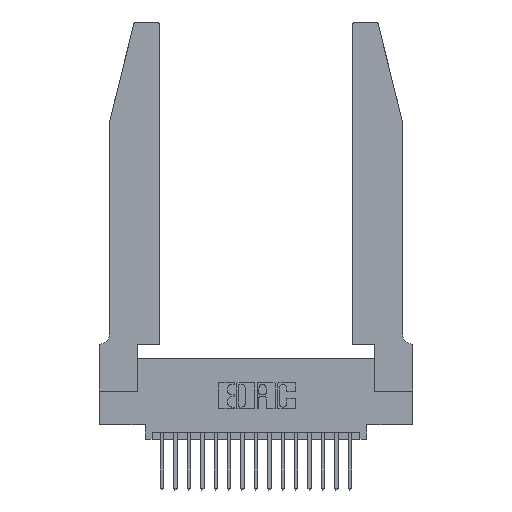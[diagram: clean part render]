
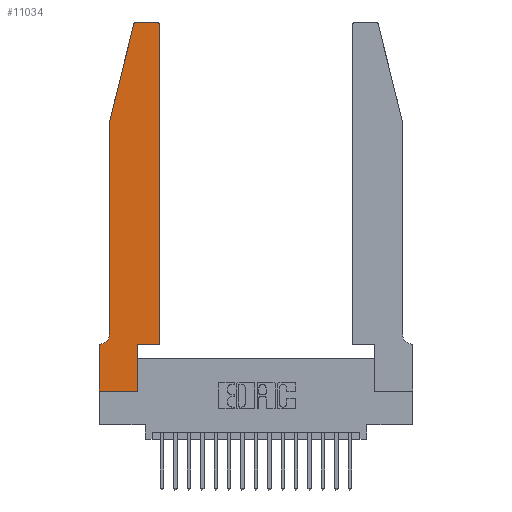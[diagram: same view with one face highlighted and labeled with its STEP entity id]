
A CAD part, top view. The second image highlights one B-rep face of the part: STEP entity #11034.
In plain terms, the highlighted planar face has unit normal (0, 0, 1).
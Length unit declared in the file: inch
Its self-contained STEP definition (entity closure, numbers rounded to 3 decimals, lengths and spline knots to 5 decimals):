
#101 = VERTEX_POINT ( 'NONE', #10746 ) ;
#145 = CARTESIAN_POINT ( 'NONE',  ( 0.4505, 2.72, 0.37 ) ) ;
#153 = ORIENTED_EDGE ( 'NONE', *, *, #16414, .T. ) ;
#239 = DIRECTION ( 'NONE',  ( -0.239, -0.971, 0. ) ) ;
#308 = DIRECTION ( 'NONE',  ( 0., 0., 1. ) ) ;
#539 = VECTOR ( 'NONE', #10012, 39.37008 ) ;
#1547 = ORIENTED_EDGE ( 'NONE', *, *, #12111, .T. ) ;
#1952 = CARTESIAN_POINT ( 'NONE',  ( 0.4505, 0.35, 0.37 ) ) ;
#1962 = VERTEX_POINT ( 'NONE', #7361 ) ;
#2054 = CIRCLE ( 'NONE', #19312, 0.03 ) ;
#2263 = DIRECTION ( 'NONE',  ( -1., 0., 0. ) ) ;
#2495 = LINE ( 'NONE', #17191, #10495 ) ;
#2787 = VECTOR ( 'NONE', #11345, 39.37008 ) ;
#3312 = LINE ( 'NONE', #6693, #2787 ) ;
#3370 = FACE_OUTER_BOUND ( 'NONE', #5832, .T. ) ;
#3449 = CIRCLE ( 'NONE', #17180, 0.07 ) ;
#3873 = EDGE_CURVE ( 'NONE', #7588, #11189, #2495, .T. ) ;
#3948 = ORIENTED_EDGE ( 'NONE', *, *, #14976, .T. ) ;
#4078 = VERTEX_POINT ( 'NONE', #8341 ) ;
#4102 = EDGE_CURVE ( 'NONE', #9212, #4964, #17397, .T. ) ;
#4835 = AXIS2_PLACEMENT_3D ( 'NONE', #15529, #17072, #7827 ) ;
#4964 = VERTEX_POINT ( 'NONE', #13429 ) ;
#5278 = VERTEX_POINT ( 'NONE', #145 ) ;
#5389 = CARTESIAN_POINT ( 'NONE',  ( 0.4505, 0.35, 0.37 ) ) ;
#5608 = CARTESIAN_POINT ( 'NONE',  ( 0.0755, 0.35, 0.37 ) ) ;
#5832 = EDGE_LOOP ( 'NONE', ( #7102, #153, #7049, #10660, #3948, #7338, #12381, #1547, #9875, #10786, #15272, #8742 ) ) ;
#5968 = VECTOR ( 'NONE', #2263, 39.37008 ) ;
#6265 = PLANE ( 'NONE',  #4835 ) ;
#6290 = VERTEX_POINT ( 'NONE', #16852 ) ;
#6476 = LINE ( 'NONE', #5608, #5968 ) ;
#6651 = CARTESIAN_POINT ( 'NONE',  ( 0.284, 2.72, 0.37 ) ) ;
#6693 = CARTESIAN_POINT ( 'NONE',  ( 0.2605, 2.75, 0.37 ) ) ;
#6741 = CIRCLE ( 'NONE', #8019, 0.03 ) ;
#7032 = DIRECTION ( 'NONE',  ( 1., 0., 0. ) ) ;
#7049 = ORIENTED_EDGE ( 'NONE', *, *, #9142, .T. ) ;
#7102 = ORIENTED_EDGE ( 'NONE', *, *, #12440, .T. ) ;
#7338 = ORIENTED_EDGE ( 'NONE', *, *, #10852, .T. ) ;
#7361 = CARTESIAN_POINT ( 'NONE',  ( 0.4205, 2.75, 0.37 ) ) ;
#7459 = DIRECTION ( 'NONE',  ( 1., 0., 0. ) ) ;
#7588 = VERTEX_POINT ( 'NONE', #9955 ) ;
#7590 = CARTESIAN_POINT ( 'NONE',  ( 0.0055, 0.42, 0.37 ) ) ;
#7827 = DIRECTION ( 'NONE',  ( 1., 0., 0. ) ) ;
#7936 = VECTOR ( 'NONE', #7032, 39.37008 ) ;
#8019 = AXIS2_PLACEMENT_3D ( 'NONE', #6651, #17466, #8211 ) ;
#8211 = DIRECTION ( 'NONE',  ( 1., 0., 0. ) ) ;
#8341 = CARTESIAN_POINT ( 'NONE',  ( 0.0055, 0.35, 0.37 ) ) ;
#8392 = CARTESIAN_POINT ( 'NONE',  ( 0.0755, 2., 0.37 ) ) ;
#8549 = EDGE_CURVE ( 'NONE', #16070, #5278, #16534, .T. ) ;
#8742 = ORIENTED_EDGE ( 'NONE', *, *, #19564, .T. ) ;
#8851 = LINE ( 'NONE', #11962, #16584 ) ;
#8934 = EDGE_CURVE ( 'NONE', #14857, #16331, #16998, .T. ) ;
#9135 = DIRECTION ( 'NONE',  ( -1., 0., 0. ) ) ;
#9142 = EDGE_CURVE ( 'NONE', #6290, #14857, #18186, .T. ) ;
#9212 = VERTEX_POINT ( 'NONE', #19320 ) ;
#9424 = CARTESIAN_POINT ( 'NONE',  ( 0.0755, 0.42, 0.37 ) ) ;
#9875 = ORIENTED_EDGE ( 'NONE', *, *, #4102, .T. ) ;
#9955 = CARTESIAN_POINT ( 'NONE',  ( 0., 0.35, 0.37 ) ) ;
#9995 = CARTESIAN_POINT ( 'NONE',  ( 0.4205, 2.72, 0.37 ) ) ;
#10012 = DIRECTION ( 'NONE',  ( 0., 1., 0. ) ) ;
#10308 = CARTESIAN_POINT ( 'NONE',  ( 0.4505, 0.35, 0.37 ) ) ;
#10495 = VECTOR ( 'NONE', #18685, 39.37008 ) ;
#10660 = ORIENTED_EDGE ( 'NONE', *, *, #8934, .T. ) ;
#10746 = CARTESIAN_POINT ( 'NONE',  ( 0.284, 2.75, 0.37 ) ) ;
#10765 = EDGE_CURVE ( 'NONE', #4964, #16070, #12025, .T. ) ;
#10786 = ORIENTED_EDGE ( 'NONE', *, *, #10765, .T. ) ;
#10852 = EDGE_CURVE ( 'NONE', #4078, #7588, #6476, .T. ) ;
#11034 = ADVANCED_FACE ( 'NONE', ( #3370 ), #6265, .T. ) ;
#11189 = VERTEX_POINT ( 'NONE', #12735 ) ;
#11345 = DIRECTION ( 'NONE',  ( -1., 0., 0. ) ) ;
#11552 = DIRECTION ( 'NONE',  ( 1., 0., 0. ) ) ;
#11927 = VECTOR ( 'NONE', #14642, 39.37008 ) ;
#11962 = CARTESIAN_POINT ( 'NONE',  ( 0., 0., 0.37 ) ) ;
#12025 = LINE ( 'NONE', #5389, #7936 ) ;
#12111 = EDGE_CURVE ( 'NONE', #11189, #9212, #8851, .T. ) ;
#12381 = ORIENTED_EDGE ( 'NONE', *, *, #3873, .T. ) ;
#12440 = EDGE_CURVE ( 'NONE', #1962, #101, #3312, .T. ) ;
#12735 = CARTESIAN_POINT ( 'NONE',  ( 0., 0., 0.37 ) ) ;
#12876 = VECTOR ( 'NONE', #17248, 39.37008 ) ;
#13382 = CARTESIAN_POINT ( 'NONE',  ( 0.0755, 2., 0.37 ) ) ;
#13429 = CARTESIAN_POINT ( 'NONE',  ( 0.2865, 0.35, 0.37 ) ) ;
#14076 = VECTOR ( 'NONE', #239, 39.37008 ) ;
#14135 = CARTESIAN_POINT ( 'NONE',  ( 0.0755, 2., 0.37 ) ) ;
#14642 = DIRECTION ( 'NONE',  ( 0., 1., 0. ) ) ;
#14857 = VERTEX_POINT ( 'NONE', #13382 ) ;
#14976 = EDGE_CURVE ( 'NONE', #16331, #4078, #3449, .T. ) ;
#15272 = ORIENTED_EDGE ( 'NONE', *, *, #8549, .T. ) ;
#15529 = CARTESIAN_POINT ( 'NONE',  ( 0., 0.35, 0.37 ) ) ;
#16070 = VERTEX_POINT ( 'NONE', #10308 ) ;
#16331 = VERTEX_POINT ( 'NONE', #9424 ) ;
#16414 = EDGE_CURVE ( 'NONE', #101, #6290, #6741, .T. ) ;
#16534 = LINE ( 'NONE', #1952, #11927 ) ;
#16584 = VECTOR ( 'NONE', #7459, 39.37008 ) ;
#16852 = CARTESIAN_POINT ( 'NONE',  ( 0.25487, 2.72718, 0.37 ) ) ;
#16998 = LINE ( 'NONE', #14135, #12876 ) ;
#17072 = DIRECTION ( 'NONE',  ( 0., 0., 1. ) ) ;
#17180 = AXIS2_PLACEMENT_3D ( 'NONE', #7590, #18353, #9135 ) ;
#17191 = CARTESIAN_POINT ( 'NONE',  ( 0., 0., 0.37 ) ) ;
#17248 = DIRECTION ( 'NONE',  ( 0., -1., 0. ) ) ;
#17397 = LINE ( 'NONE', #17726, #539 ) ;
#17466 = DIRECTION ( 'NONE',  ( 0., 0., 1. ) ) ;
#17726 = CARTESIAN_POINT ( 'NONE',  ( 0.2865, 0.35, 0.37 ) ) ;
#18186 = LINE ( 'NONE', #8392, #14076 ) ;
#18353 = DIRECTION ( 'NONE',  ( 0., 0., -1. ) ) ;
#18685 = DIRECTION ( 'NONE',  ( 0., -1., 0. ) ) ;
#19312 = AXIS2_PLACEMENT_3D ( 'NONE', #9995, #308, #11552 ) ;
#19320 = CARTESIAN_POINT ( 'NONE',  ( 0.2865, 0., 0.37 ) ) ;
#19564 = EDGE_CURVE ( 'NONE', #5278, #1962, #2054, .T. ) ;
